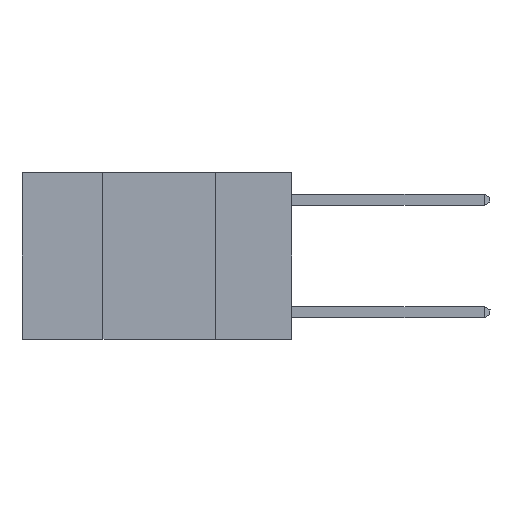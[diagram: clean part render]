
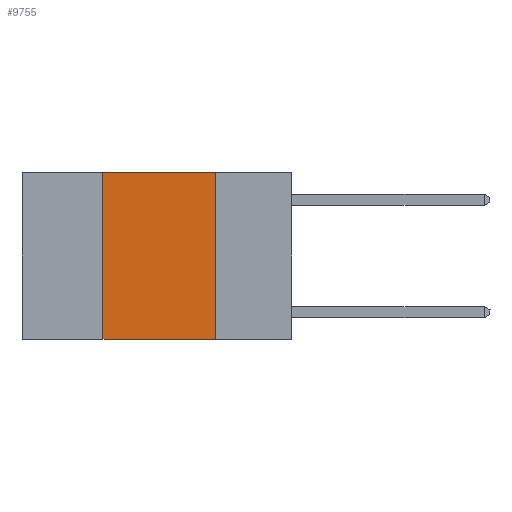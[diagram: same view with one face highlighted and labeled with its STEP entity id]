
A CAD part, left-side view. The second image highlights one B-rep face of the part: STEP entity #9755.
In plain terms, the highlighted planar face has unit normal (-1, 0, 0).
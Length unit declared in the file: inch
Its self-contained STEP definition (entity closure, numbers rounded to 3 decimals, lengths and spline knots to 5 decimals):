
#335 = LINE ( 'NONE', #347, #571 ) ;
#347 = CARTESIAN_POINT ( 'NONE',  ( 0., 0.6, 0. ) ) ;
#479 = VERTEX_POINT ( 'NONE', #8113 ) ;
#571 = VECTOR ( 'NONE', #5949, 39.37008 ) ;
#574 = CARTESIAN_POINT ( 'NONE',  ( 0., 0.6, -0.37 ) ) ;
#625 = ORIENTED_EDGE ( 'NONE', *, *, #7611, .F. ) ;
#977 = VECTOR ( 'NONE', #9416, 39.37008 ) ;
#1321 = DIRECTION ( 'NONE',  ( 0., -1., 0. ) ) ;
#1363 = DIRECTION ( 'NONE',  ( 0., 0., 1. ) ) ;
#1371 = VECTOR ( 'NONE', #1363, 39.37008 ) ;
#1638 = PLANE ( 'NONE',  #1973 ) ;
#1973 = AXIS2_PLACEMENT_3D ( 'NONE', #8836, #4083, #9621 ) ;
#2487 = EDGE_CURVE ( 'NONE', #6523, #6660, #7367, .T. ) ;
#3159 = VECTOR ( 'NONE', #1321, 39.37008 ) ;
#3757 = EDGE_CURVE ( 'NONE', #9324, #479, #335, .T. ) ;
#4083 = DIRECTION ( 'NONE',  ( 1., 0., 0. ) ) ;
#4115 = CARTESIAN_POINT ( 'NONE',  ( 0., 0.42, -0.37 ) ) ;
#4858 = ORIENTED_EDGE ( 'NONE', *, *, #2487, .T. ) ;
#5022 = CARTESIAN_POINT ( 'NONE',  ( 0., 0.42, 0. ) ) ;
#5238 = LINE ( 'NONE', #8650, #977 ) ;
#5615 = ORIENTED_EDGE ( 'NONE', *, *, #3757, .F. ) ;
#5949 = DIRECTION ( 'NONE',  ( 0., -1., 0. ) ) ;
#6523 = VERTEX_POINT ( 'NONE', #4115 ) ;
#6660 = VERTEX_POINT ( 'NONE', #8221 ) ;
#6899 = EDGE_LOOP ( 'NONE', ( #7710, #5615, #625, #4858 ) ) ;
#7367 = LINE ( 'NONE', #574, #3159 ) ;
#7611 = EDGE_CURVE ( 'NONE', #6523, #9324, #7753, .T. ) ;
#7710 = ORIENTED_EDGE ( 'NONE', *, *, #8758, .F. ) ;
#7753 = LINE ( 'NONE', #9294, #1371 ) ;
#8113 = CARTESIAN_POINT ( 'NONE',  ( 0., 0.17, 0. ) ) ;
#8221 = CARTESIAN_POINT ( 'NONE',  ( 0., 0.17, -0.37 ) ) ;
#8650 = CARTESIAN_POINT ( 'NONE',  ( 0., 0.17, 0. ) ) ;
#8758 = EDGE_CURVE ( 'NONE', #479, #6660, #5238, .T. ) ;
#8836 = CARTESIAN_POINT ( 'NONE',  ( 0., 0.6, 0. ) ) ;
#9289 = FACE_OUTER_BOUND ( 'NONE', #6899, .T. ) ;
#9294 = CARTESIAN_POINT ( 'NONE',  ( 0., 0.42, 0. ) ) ;
#9324 = VERTEX_POINT ( 'NONE', #5022 ) ;
#9416 = DIRECTION ( 'NONE',  ( 0., 0., -1. ) ) ;
#9621 = DIRECTION ( 'NONE',  ( 0., 0., -1. ) ) ;
#9755 = ADVANCED_FACE ( 'NONE', ( #9289 ), #1638, .F. ) ;
